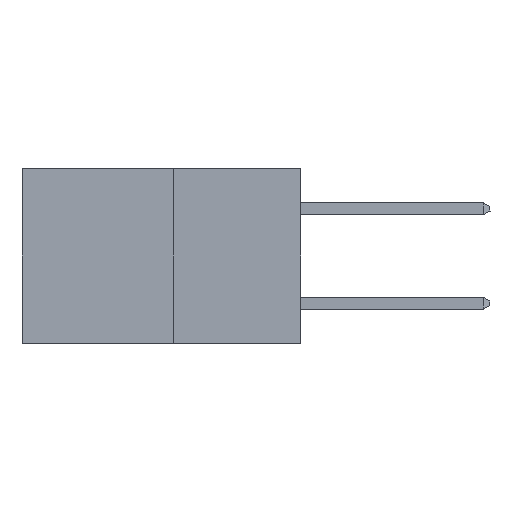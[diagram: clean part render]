
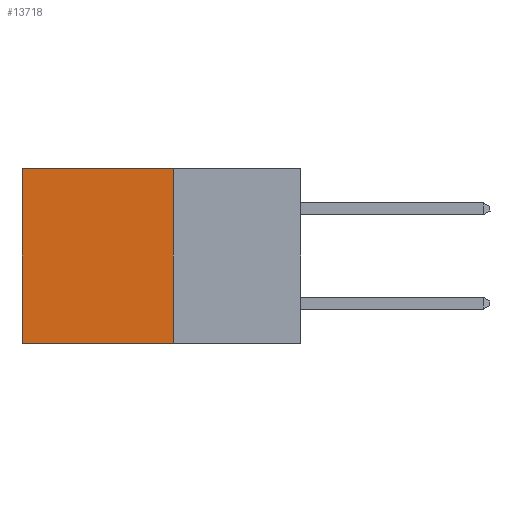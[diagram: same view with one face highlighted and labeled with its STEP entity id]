
A CAD part, left-side view. The second image highlights one B-rep face of the part: STEP entity #13718.
In plain terms, the highlighted planar face has unit normal (-1, 0, 0).
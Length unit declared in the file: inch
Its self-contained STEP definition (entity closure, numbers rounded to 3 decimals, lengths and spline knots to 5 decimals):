
#445 = LINE ( 'NONE', #1842, #6203 ) ;
#1713 = CARTESIAN_POINT ( 'NONE',  ( 0.277, 0.59, 0. ) ) ;
#1842 = CARTESIAN_POINT ( 'NONE',  ( 0.277, 0.27, 0. ) ) ;
#2096 = VECTOR ( 'NONE', #7968, 39.37008 ) ;
#2351 = CARTESIAN_POINT ( 'NONE',  ( 0.277, 0.59, -0.37 ) ) ;
#2703 = VECTOR ( 'NONE', #13146, 39.37008 ) ;
#2759 = PLANE ( 'NONE',  #4711 ) ;
#2853 = ORIENTED_EDGE ( 'NONE', *, *, #13497, .T. ) ;
#2869 = EDGE_CURVE ( 'NONE', #10177, #13498, #5775, .T. ) ;
#3916 = DIRECTION ( 'NONE',  ( 0., 0., -1. ) ) ;
#4566 = ORIENTED_EDGE ( 'NONE', *, *, #7594, .F. ) ;
#4711 = AXIS2_PLACEMENT_3D ( 'NONE', #12780, #10510, #3916 ) ;
#4724 = CARTESIAN_POINT ( 'NONE',  ( 0.277, 0.59, -0.37 ) ) ;
#5766 = EDGE_LOOP ( 'NONE', ( #2853, #11256, #4566, #13075 ) ) ;
#5775 = LINE ( 'NONE', #8631, #2703 ) ;
#6203 = VECTOR ( 'NONE', #9617, 39.37008 ) ;
#6515 = VERTEX_POINT ( 'NONE', #8179 ) ;
#7594 = EDGE_CURVE ( 'NONE', #6515, #10177, #8185, .T. ) ;
#7915 = FACE_OUTER_BOUND ( 'NONE', #5766, .T. ) ;
#7968 = DIRECTION ( 'NONE',  ( 0., 0., -1. ) ) ;
#8179 = CARTESIAN_POINT ( 'NONE',  ( 0.277, 0.27, 0. ) ) ;
#8185 = LINE ( 'NONE', #9997, #13803 ) ;
#8631 = CARTESIAN_POINT ( 'NONE',  ( 0.277, 0.27, -0.37 ) ) ;
#9617 = DIRECTION ( 'NONE',  ( 0., 1., 0. ) ) ;
#9961 = DIRECTION ( 'NONE',  ( 0., 0., -1. ) ) ;
#9997 = CARTESIAN_POINT ( 'NONE',  ( 0.277, 0.27, -0.37 ) ) ;
#10177 = VERTEX_POINT ( 'NONE', #13198 ) ;
#10510 = DIRECTION ( 'NONE',  ( 1., 0., 0. ) ) ;
#10997 = LINE ( 'NONE', #2351, #2096 ) ;
#11256 = ORIENTED_EDGE ( 'NONE', *, *, #2869, .F. ) ;
#12780 = CARTESIAN_POINT ( 'NONE',  ( 0.277, 0.27, -0.37 ) ) ;
#13075 = ORIENTED_EDGE ( 'NONE', *, *, #13853, .T. ) ;
#13091 = VERTEX_POINT ( 'NONE', #1713 ) ;
#13146 = DIRECTION ( 'NONE',  ( 0., 1., 0. ) ) ;
#13198 = CARTESIAN_POINT ( 'NONE',  ( 0.277, 0.27, -0.37 ) ) ;
#13497 = EDGE_CURVE ( 'NONE', #13091, #13498, #10997, .T. ) ;
#13498 = VERTEX_POINT ( 'NONE', #4724 ) ;
#13718 = ADVANCED_FACE ( 'NONE', ( #7915 ), #2759, .F. ) ;
#13803 = VECTOR ( 'NONE', #9961, 39.37008 ) ;
#13853 = EDGE_CURVE ( 'NONE', #6515, #13091, #445, .T. ) ;
